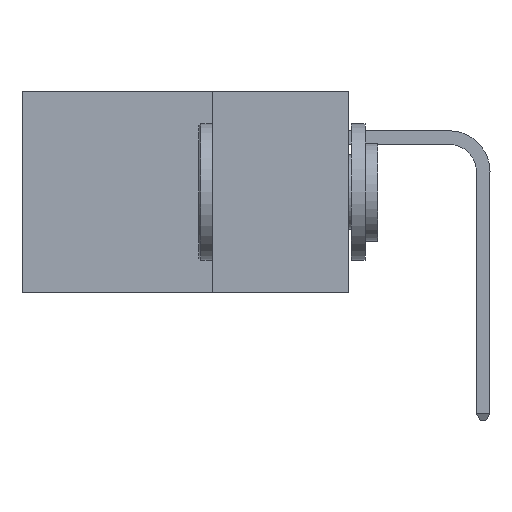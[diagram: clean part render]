
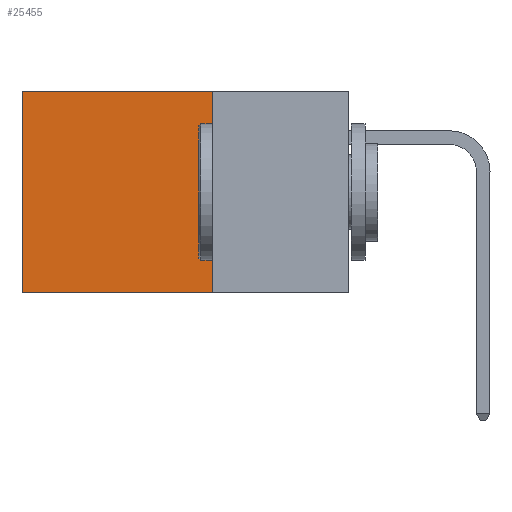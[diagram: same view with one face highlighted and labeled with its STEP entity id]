
A CAD part, left-side view. The second image highlights one B-rep face of the part: STEP entity #25455.
In plain terms, the highlighted planar face has unit normal (-1, 0, 0).
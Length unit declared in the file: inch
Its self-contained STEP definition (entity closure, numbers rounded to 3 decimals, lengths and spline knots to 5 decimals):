
#1914 = PLANE ( 'NONE',  #5932 ) ;
#3570 = VECTOR ( 'NONE', #15098, 39.37008 ) ;
#3784 = VERTEX_POINT ( 'NONE', #16846 ) ;
#5193 = CARTESIAN_POINT ( 'NONE',  ( 0.2875, 0.6, 0. ) ) ;
#5932 = AXIS2_PLACEMENT_3D ( 'NONE', #7773, #34038, #16635 ) ;
#6500 = ORIENTED_EDGE ( 'NONE', *, *, #16187, .T. ) ;
#7773 = CARTESIAN_POINT ( 'NONE',  ( 0.2875, 0.25, 0. ) ) ;
#10348 = CARTESIAN_POINT ( 'NONE',  ( 0.2875, 0.25, -0.37 ) ) ;
#10872 = EDGE_LOOP ( 'NONE', ( #6500, #20665, #16662, #28205 ) ) ;
#15098 = DIRECTION ( 'NONE',  ( 0., 0., -1. ) ) ;
#15545 = VERTEX_POINT ( 'NONE', #32572 ) ;
#16187 = EDGE_CURVE ( 'NONE', #23610, #3784, #34573, .T. ) ;
#16635 = DIRECTION ( 'NONE',  ( 0., 0., -1. ) ) ;
#16662 = ORIENTED_EDGE ( 'NONE', *, *, #36816, .F. ) ;
#16755 = CARTESIAN_POINT ( 'NONE',  ( 0.2875, 0.25, 0. ) ) ;
#16846 = CARTESIAN_POINT ( 'NONE',  ( 0.2875, 0.6, -0.37 ) ) ;
#17146 = VERTEX_POINT ( 'NONE', #25343 ) ;
#18527 = LINE ( 'NONE', #16755, #35799 ) ;
#20665 = ORIENTED_EDGE ( 'NONE', *, *, #36453, .F. ) ;
#21110 = DIRECTION ( 'NONE',  ( 0., 1., 0. ) ) ;
#23555 = VECTOR ( 'NONE', #30749, 39.37008 ) ;
#23610 = VERTEX_POINT ( 'NONE', #5193 ) ;
#25343 = CARTESIAN_POINT ( 'NONE',  ( 0.2875, 0.25, -0.37 ) ) ;
#25455 = ADVANCED_FACE ( 'NONE', ( #28564 ), #1914, .F. ) ;
#26795 = VECTOR ( 'NONE', #21110, 39.37008 ) ;
#28205 = ORIENTED_EDGE ( 'NONE', *, *, #35764, .T. ) ;
#28287 = DIRECTION ( 'NONE',  ( 0., 0., -1. ) ) ;
#28564 = FACE_OUTER_BOUND ( 'NONE', #10872, .T. ) ;
#29768 = CARTESIAN_POINT ( 'NONE',  ( 0.2875, 0.25, 0. ) ) ;
#30373 = LINE ( 'NONE', #10348, #23555 ) ;
#30749 = DIRECTION ( 'NONE',  ( 0., 1., 0. ) ) ;
#32572 = CARTESIAN_POINT ( 'NONE',  ( 0.2875, 0.25, 0. ) ) ;
#34038 = DIRECTION ( 'NONE',  ( 1., 0., 0. ) ) ;
#34535 = LINE ( 'NONE', #29768, #26795 ) ;
#34573 = LINE ( 'NONE', #35432, #3570 ) ;
#35432 = CARTESIAN_POINT ( 'NONE',  ( 0.2875, 0.6, 0. ) ) ;
#35764 = EDGE_CURVE ( 'NONE', #15545, #23610, #34535, .T. ) ;
#35799 = VECTOR ( 'NONE', #28287, 39.37008 ) ;
#36453 = EDGE_CURVE ( 'NONE', #17146, #3784, #30373, .T. ) ;
#36816 = EDGE_CURVE ( 'NONE', #15545, #17146, #18527, .T. ) ;
